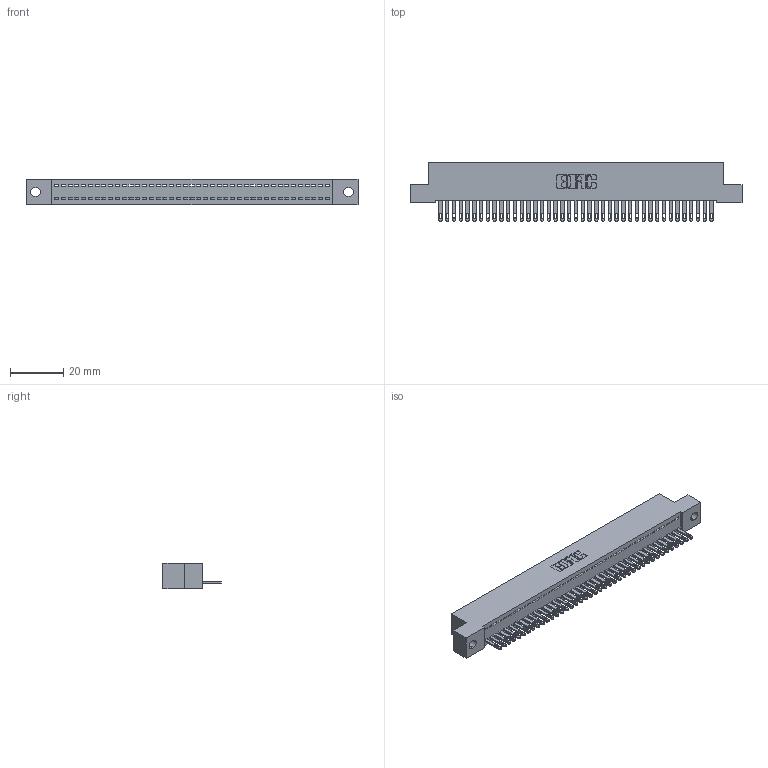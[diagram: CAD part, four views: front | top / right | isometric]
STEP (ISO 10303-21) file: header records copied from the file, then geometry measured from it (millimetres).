
FILE_DESCRIPTION (( 'STEP AP203' ), '1' );
FILE_NAME ('892-041-500-102.STEP', '2020-09-21T16:32:39', ( '' ), ( '' ), 'SwSTEP 2.0', 'SolidWorks 2020', '' );
FILE_SCHEMA (( 'CONFIG_CONTROL_DESIGN' ));
Length unit declared in the file: inch
Products named in the file (3): 842 Part_.128 Slot; 892-041-500-102; 345-292-001_345-293-100
Assembly tree (42 placements, depth 2):
  892-041-500-102
    842 Part_.128 Slot
    345-292-001_345-293-100  x41
Bounding box: 124.46 x 21.85 x 9.4 mm (x, y, z)
Volume: 10882.2 mm3; surface area: 15801.7 mm2
Topology: 42 solids, 42 shells, 2328 faces, 7199 edges, 4798 vertices
Faces by surface type: plane 1546, cylinder 782
Entity records: 25127 total; most frequent: CARTESIAN_POINT 4341, ORIENTED_EDGE 4318, DIRECTION 3665, EDGE_CURVE 2159, LINE 2027, VECTOR 2027, VERTEX_POINT 1438, AXIS2_PLACEMENT_3D 819
